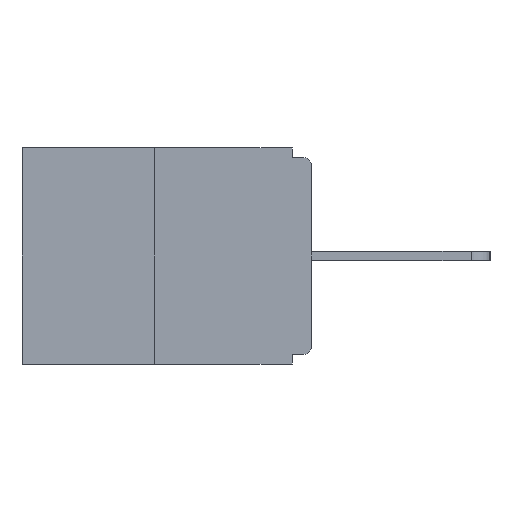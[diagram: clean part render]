
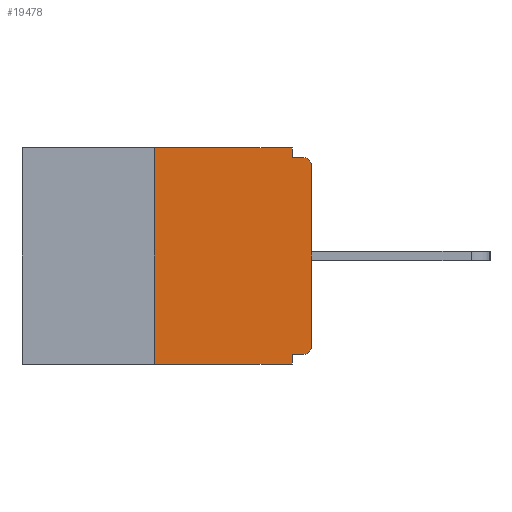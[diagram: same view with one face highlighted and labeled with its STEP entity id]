
A CAD part, left-side view. The second image highlights one B-rep face of the part: STEP entity #19478.
In plain terms, the highlighted planar face has unit normal (-1, 0, 0).
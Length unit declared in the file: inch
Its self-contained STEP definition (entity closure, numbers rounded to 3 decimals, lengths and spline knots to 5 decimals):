
#144 = DIRECTION ( 'NONE',  ( 0., 0., -1. ) ) ;
#208 = CARTESIAN_POINT ( 'NONE',  ( 0., 0.015, -0.03 ) ) ;
#249 = LINE ( 'NONE', #479, #10407 ) ;
#479 = CARTESIAN_POINT ( 'NONE',  ( 0., 0.031, 0. ) ) ;
#1485 = VECTOR ( 'NONE', #10830, 39.37008 ) ;
#1784 = EDGE_CURVE ( 'NONE', #16420, #2360, #3523, .T. ) ;
#2360 = VERTEX_POINT ( 'NONE', #12451 ) ;
#3523 = LINE ( 'NONE', #8241, #14798 ) ;
#3856 = LINE ( 'NONE', #13950, #1485 ) ;
#4062 = ORIENTED_EDGE ( 'NONE', *, *, #11768, .F. ) ;
#4192 = EDGE_CURVE ( 'NONE', #17350, #15652, #11415, .T. ) ;
#4622 = CIRCLE ( 'NONE', #9265, 0.015 ) ;
#5147 = DIRECTION ( 'NONE',  ( 1., 0., 0. ) ) ;
#5542 = LINE ( 'NONE', #9011, #7469 ) ;
#5673 = DIRECTION ( 'NONE',  ( 0., 0., -1. ) ) ;
#6062 = ORIENTED_EDGE ( 'NONE', *, *, #9397, .F. ) ;
#6135 = CARTESIAN_POINT ( 'NONE',  ( 0., 0.015, -0.328 ) ) ;
#6450 = ORIENTED_EDGE ( 'NONE', *, *, #18889, .T. ) ;
#6928 = ORIENTED_EDGE ( 'NONE', *, *, #12414, .F. ) ;
#7041 = VERTEX_POINT ( 'NONE', #9491 ) ;
#7269 = EDGE_CURVE ( 'NONE', #7041, #11386, #5542, .T. ) ;
#7469 = VECTOR ( 'NONE', #10820, 39.37008 ) ;
#7584 = AXIS2_PLACEMENT_3D ( 'NONE', #208, #9456, #15750 ) ;
#7917 = DIRECTION ( 'NONE',  ( 0., 0., 1. ) ) ;
#7935 = CIRCLE ( 'NONE', #7584, 0.015 ) ;
#8054 = EDGE_CURVE ( 'NONE', #11672, #16420, #4622, .T. ) ;
#8241 = CARTESIAN_POINT ( 'NONE',  ( 0., 0., 0. ) ) ;
#8252 = LINE ( 'NONE', #21774, #19268 ) ;
#8258 = VECTOR ( 'NONE', #15920, 39.37008 ) ;
#8454 = DIRECTION ( 'NONE',  ( 0., 0., 1. ) ) ;
#8941 = CARTESIAN_POINT ( 'NONE',  ( 0., 0.25, 0. ) ) ;
#9011 = CARTESIAN_POINT ( 'NONE',  ( 0., 0.46, -0.343 ) ) ;
#9265 = AXIS2_PLACEMENT_3D ( 'NONE', #19439, #13973, #5673 ) ;
#9397 = EDGE_CURVE ( 'NONE', #13883, #17350, #249, .T. ) ;
#9456 = DIRECTION ( 'NONE',  ( -1., 0., 0. ) ) ;
#9491 = CARTESIAN_POINT ( 'NONE',  ( 0., 0.25, -0.343 ) ) ;
#9583 = VERTEX_POINT ( 'NONE', #18853 ) ;
#9789 = EDGE_CURVE ( 'NONE', #9583, #11386, #3856, .T. ) ;
#9840 = ORIENTED_EDGE ( 'NONE', *, *, #9789, .F. ) ;
#10220 = CARTESIAN_POINT ( 'NONE',  ( 0., 0.031, -0.015 ) ) ;
#10407 = VECTOR ( 'NONE', #144, 39.37008 ) ;
#10820 = DIRECTION ( 'NONE',  ( 0., -1., 0. ) ) ;
#10830 = DIRECTION ( 'NONE',  ( 0., 0., -1. ) ) ;
#11290 = ORIENTED_EDGE ( 'NONE', *, *, #1784, .T. ) ;
#11386 = VERTEX_POINT ( 'NONE', #21708 ) ;
#11407 = CARTESIAN_POINT ( 'NONE',  ( 0., 0., -0.328 ) ) ;
#11415 = LINE ( 'NONE', #18214, #8258 ) ;
#11606 = CARTESIAN_POINT ( 'NONE',  ( 0., 0.015, -0.015 ) ) ;
#11672 = VERTEX_POINT ( 'NONE', #6135 ) ;
#11764 = PLANE ( 'NONE',  #18683 ) ;
#11768 = EDGE_CURVE ( 'NONE', #7041, #19692, #8252, .T. ) ;
#12414 = EDGE_CURVE ( 'NONE', #19692, #13883, #16039, .T. ) ;
#12451 = CARTESIAN_POINT ( 'NONE',  ( 0., 0., -0.03 ) ) ;
#12664 = ORIENTED_EDGE ( 'NONE', *, *, #7269, .T. ) ;
#12742 = CARTESIAN_POINT ( 'NONE',  ( 0., 0., -0.313 ) ) ;
#13883 = VERTEX_POINT ( 'NONE', #19827 ) ;
#13950 = CARTESIAN_POINT ( 'NONE',  ( 0., 0.031, -0.343 ) ) ;
#13973 = DIRECTION ( 'NONE',  ( -1., 0., 0. ) ) ;
#14282 = VECTOR ( 'NONE', #15708, 39.37008 ) ;
#14762 = LINE ( 'NONE', #11407, #16495 ) ;
#14798 = VECTOR ( 'NONE', #8454, 39.37008 ) ;
#15652 = VERTEX_POINT ( 'NONE', #11606 ) ;
#15708 = DIRECTION ( 'NONE',  ( 0., -1., 0. ) ) ;
#15750 = DIRECTION ( 'NONE',  ( 0., 0., -1. ) ) ;
#15920 = DIRECTION ( 'NONE',  ( 0., -1., 0. ) ) ;
#16039 = LINE ( 'NONE', #21280, #14282 ) ;
#16420 = VERTEX_POINT ( 'NONE', #12742 ) ;
#16495 = VECTOR ( 'NONE', #16542, 39.37008 ) ;
#16542 = DIRECTION ( 'NONE',  ( 0., 1., 0. ) ) ;
#17004 = DIRECTION ( 'NONE',  ( 0., 0., -1. ) ) ;
#17350 = VERTEX_POINT ( 'NONE', #10220 ) ;
#18090 = ORIENTED_EDGE ( 'NONE', *, *, #18189, .F. ) ;
#18189 = EDGE_CURVE ( 'NONE', #11672, #9583, #14762, .T. ) ;
#18214 = CARTESIAN_POINT ( 'NONE',  ( 0., 0., -0.015 ) ) ;
#18258 = ORIENTED_EDGE ( 'NONE', *, *, #4192, .F. ) ;
#18683 = AXIS2_PLACEMENT_3D ( 'NONE', #20465, #5147, #17004 ) ;
#18853 = CARTESIAN_POINT ( 'NONE',  ( 0., 0.031, -0.328 ) ) ;
#18888 = FACE_OUTER_BOUND ( 'NONE', #20942, .T. ) ;
#18889 = EDGE_CURVE ( 'NONE', #2360, #15652, #7935, .T. ) ;
#19268 = VECTOR ( 'NONE', #7917, 39.37008 ) ;
#19439 = CARTESIAN_POINT ( 'NONE',  ( 0., 0.015, -0.313 ) ) ;
#19478 = ADVANCED_FACE ( 'NONE', ( #18888 ), #11764, .F. ) ;
#19692 = VERTEX_POINT ( 'NONE', #8941 ) ;
#19827 = CARTESIAN_POINT ( 'NONE',  ( 0., 0.031, 0. ) ) ;
#20465 = CARTESIAN_POINT ( 'NONE',  ( 0., 0.46, 0. ) ) ;
#20942 = EDGE_LOOP ( 'NONE', ( #6928, #4062, #12664, #9840, #18090, #21007, #11290, #6450, #18258, #6062 ) ) ;
#21007 = ORIENTED_EDGE ( 'NONE', *, *, #8054, .T. ) ;
#21280 = CARTESIAN_POINT ( 'NONE',  ( 0., 0.46, 0. ) ) ;
#21708 = CARTESIAN_POINT ( 'NONE',  ( 0., 0.031, -0.343 ) ) ;
#21774 = CARTESIAN_POINT ( 'NONE',  ( 0., 0.25, 0. ) ) ;
